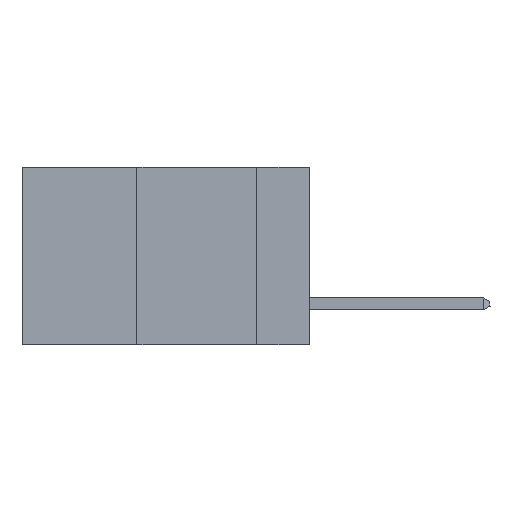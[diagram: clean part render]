
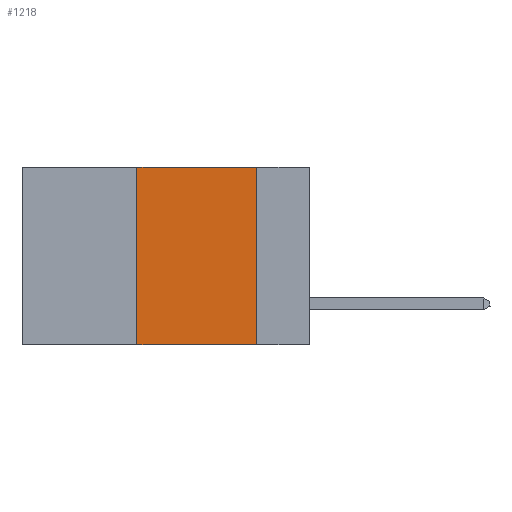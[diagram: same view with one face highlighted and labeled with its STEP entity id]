
A CAD part, left-side view. The second image highlights one B-rep face of the part: STEP entity #1218.
In plain terms, the highlighted planar face has unit normal (-1, 0, 0).
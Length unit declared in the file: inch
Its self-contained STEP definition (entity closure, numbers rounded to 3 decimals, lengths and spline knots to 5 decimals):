
#692 = DIRECTION ( 'NONE',  ( 0., 0., 1. ) ) ;
#1210 = ORIENTED_EDGE ( 'NONE', *, *, #1682, .T. ) ;
#1218 = ADVANCED_FACE ( 'NONE', ( #14907 ), #10132, .F. ) ;
#1682 = EDGE_CURVE ( 'NONE', #20758, #17158, #10466, .T. ) ;
#2486 = VECTOR ( 'NONE', #21982, 39.37008 ) ;
#2589 = VECTOR ( 'NONE', #692, 39.37008 ) ;
#3118 = CARTESIAN_POINT ( 'NONE',  ( 0., 0.11, 0. ) ) ;
#3561 = EDGE_LOOP ( 'NONE', ( #7219, #6506, #16085, #1210 ) ) ;
#3759 = DIRECTION ( 'NONE',  ( 0., -1., 0. ) ) ;
#4048 = LINE ( 'NONE', #8085, #2486 ) ;
#5714 = VECTOR ( 'NONE', #3759, 39.37008 ) ;
#6018 = VERTEX_POINT ( 'NONE', #16932 ) ;
#6208 = LINE ( 'NONE', #16640, #11236 ) ;
#6506 = ORIENTED_EDGE ( 'NONE', *, *, #15387, .F. ) ;
#7219 = ORIENTED_EDGE ( 'NONE', *, *, #19001, .F. ) ;
#7953 = DIRECTION ( 'NONE',  ( 0., 0., -1. ) ) ;
#8085 = CARTESIAN_POINT ( 'NONE',  ( 0., 0.11, 0. ) ) ;
#8221 = AXIS2_PLACEMENT_3D ( 'NONE', #22023, #14275, #7953 ) ;
#8603 = DIRECTION ( 'NONE',  ( 0., -1., 0. ) ) ;
#10132 = PLANE ( 'NONE',  #8221 ) ;
#10466 = LINE ( 'NONE', #18091, #5714 ) ;
#11236 = VECTOR ( 'NONE', #8603, 39.37008 ) ;
#12667 = CARTESIAN_POINT ( 'NONE',  ( 0., 0.11, -0.37 ) ) ;
#12949 = CARTESIAN_POINT ( 'NONE',  ( 0., 0.36, 0. ) ) ;
#14275 = DIRECTION ( 'NONE',  ( 1., 0., 0. ) ) ;
#14907 = FACE_OUTER_BOUND ( 'NONE', #3561, .T. ) ;
#15356 = CARTESIAN_POINT ( 'NONE',  ( 0., 0.36, -0.37 ) ) ;
#15387 = EDGE_CURVE ( 'NONE', #6018, #24684, #6208, .T. ) ;
#16085 = ORIENTED_EDGE ( 'NONE', *, *, #23373, .F. ) ;
#16640 = CARTESIAN_POINT ( 'NONE',  ( 0., 0.6, 0. ) ) ;
#16932 = CARTESIAN_POINT ( 'NONE',  ( 0., 0.36, 0. ) ) ;
#17158 = VERTEX_POINT ( 'NONE', #12667 ) ;
#18091 = CARTESIAN_POINT ( 'NONE',  ( 0., 0.6, -0.37 ) ) ;
#19001 = EDGE_CURVE ( 'NONE', #24684, #17158, #4048, .T. ) ;
#20758 = VERTEX_POINT ( 'NONE', #15356 ) ;
#21982 = DIRECTION ( 'NONE',  ( 0., 0., -1. ) ) ;
#22023 = CARTESIAN_POINT ( 'NONE',  ( 0., 0.6, 0. ) ) ;
#23373 = EDGE_CURVE ( 'NONE', #20758, #6018, #24124, .T. ) ;
#24124 = LINE ( 'NONE', #12949, #2589 ) ;
#24684 = VERTEX_POINT ( 'NONE', #3118 ) ;
